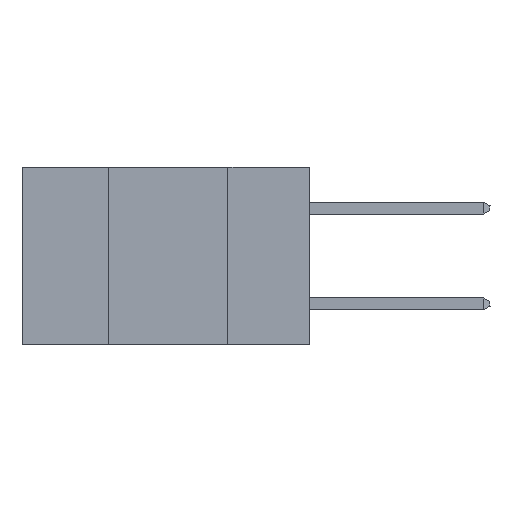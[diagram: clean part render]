
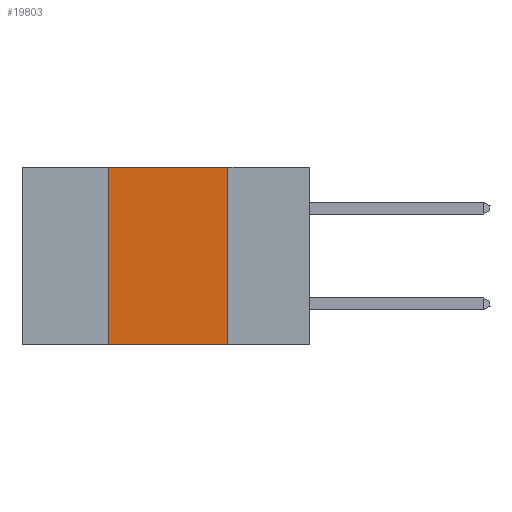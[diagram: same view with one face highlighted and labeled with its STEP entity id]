
A CAD part, left-side view. The second image highlights one B-rep face of the part: STEP entity #19803.
In plain terms, the highlighted planar face has unit normal (-1, 0, 0).
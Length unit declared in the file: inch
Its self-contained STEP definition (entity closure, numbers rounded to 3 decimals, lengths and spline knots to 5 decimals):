
#397 = DIRECTION ( 'NONE',  ( 0., 0., -1. ) ) ;
#1202 = LINE ( 'NONE', #20171, #11800 ) ;
#1266 = VERTEX_POINT ( 'NONE', #9523 ) ;
#1562 = VERTEX_POINT ( 'NONE', #2977 ) ;
#1728 = CARTESIAN_POINT ( 'NONE',  ( 0., 0.42, 0. ) ) ;
#1879 = LINE ( 'NONE', #14958, #2995 ) ;
#2372 = DIRECTION ( 'NONE',  ( 0., -1., 0. ) ) ;
#2729 = EDGE_LOOP ( 'NONE', ( #14290, #15767, #4992, #16524 ) ) ;
#2921 = DIRECTION ( 'NONE',  ( 0., -1., 0. ) ) ;
#2977 = CARTESIAN_POINT ( 'NONE',  ( 0., 0.42, -0.37 ) ) ;
#2995 = VECTOR ( 'NONE', #2921, 39.37008 ) ;
#3573 = VECTOR ( 'NONE', #9094, 39.37008 ) ;
#3755 = EDGE_CURVE ( 'NONE', #1266, #6245, #1202, .T. ) ;
#4061 = AXIS2_PLACEMENT_3D ( 'NONE', #7088, #18954, #397 ) ;
#4992 = ORIENTED_EDGE ( 'NONE', *, *, #6882, .F. ) ;
#6245 = VERTEX_POINT ( 'NONE', #11051 ) ;
#6882 = EDGE_CURVE ( 'NONE', #1562, #10218, #13915, .T. ) ;
#7088 = CARTESIAN_POINT ( 'NONE',  ( 0., 0.6, 0. ) ) ;
#7244 = CARTESIAN_POINT ( 'NONE',  ( 0., 0.42, 0. ) ) ;
#7649 = CARTESIAN_POINT ( 'NONE',  ( 0., 0.6, 0. ) ) ;
#8443 = LINE ( 'NONE', #7649, #10547 ) ;
#9094 = DIRECTION ( 'NONE',  ( 0., 0., 1. ) ) ;
#9523 = CARTESIAN_POINT ( 'NONE',  ( 0., 0.17, 0. ) ) ;
#10218 = VERTEX_POINT ( 'NONE', #1728 ) ;
#10547 = VECTOR ( 'NONE', #2372, 39.37008 ) ;
#11051 = CARTESIAN_POINT ( 'NONE',  ( 0., 0.17, -0.37 ) ) ;
#11800 = VECTOR ( 'NONE', #20098, 39.37008 ) ;
#13336 = EDGE_CURVE ( 'NONE', #1562, #6245, #1879, .T. ) ;
#13915 = LINE ( 'NONE', #7244, #3573 ) ;
#14290 = ORIENTED_EDGE ( 'NONE', *, *, #3755, .F. ) ;
#14315 = FACE_OUTER_BOUND ( 'NONE', #2729, .T. ) ;
#14958 = CARTESIAN_POINT ( 'NONE',  ( 0., 0.6, -0.37 ) ) ;
#14970 = EDGE_CURVE ( 'NONE', #10218, #1266, #8443, .T. ) ;
#15767 = ORIENTED_EDGE ( 'NONE', *, *, #14970, .F. ) ;
#16524 = ORIENTED_EDGE ( 'NONE', *, *, #13336, .T. ) ;
#17282 = PLANE ( 'NONE',  #4061 ) ;
#18954 = DIRECTION ( 'NONE',  ( 1., 0., 0. ) ) ;
#19803 = ADVANCED_FACE ( 'NONE', ( #14315 ), #17282, .F. ) ;
#20098 = DIRECTION ( 'NONE',  ( 0., 0., -1. ) ) ;
#20171 = CARTESIAN_POINT ( 'NONE',  ( 0., 0.17, 0. ) ) ;
